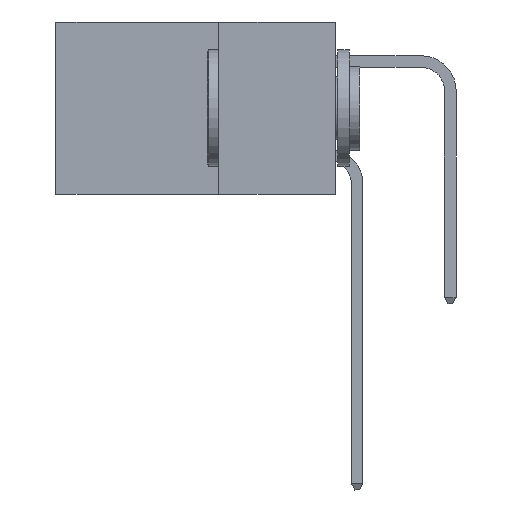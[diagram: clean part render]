
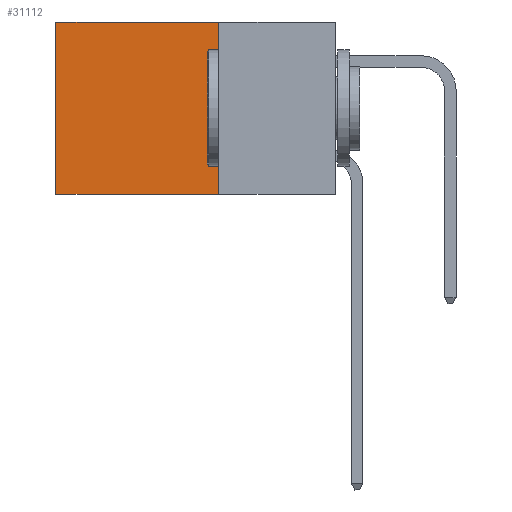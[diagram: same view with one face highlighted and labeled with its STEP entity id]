
A CAD part, left-side view. The second image highlights one B-rep face of the part: STEP entity #31112.
In plain terms, the highlighted planar face has unit normal (-1, 0, 0).
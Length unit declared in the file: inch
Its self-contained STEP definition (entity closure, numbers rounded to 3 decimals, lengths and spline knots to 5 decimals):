
#366 = DIRECTION ( 'NONE',  ( 0., 0., -1. ) ) ;
#1197 = CARTESIAN_POINT ( 'NONE',  ( 0.2875, 0.25, 0. ) ) ;
#2785 = PLANE ( 'NONE',  #10819 ) ;
#3038 = EDGE_CURVE ( 'NONE', #17193, #27264, #29164, .T. ) ;
#5011 = CARTESIAN_POINT ( 'NONE',  ( 0.2875, 0.25, -0.37 ) ) ;
#5106 = VECTOR ( 'NONE', #8847, 39.37008 ) ;
#6699 = CARTESIAN_POINT ( 'NONE',  ( 0.2875, 0.25, 0. ) ) ;
#6942 = EDGE_LOOP ( 'NONE', ( #30878, #9580, #10173, #22482 ) ) ;
#7513 = LINE ( 'NONE', #6699, #21998 ) ;
#7831 = CARTESIAN_POINT ( 'NONE',  ( 0.2875, 0.6, 0. ) ) ;
#8000 = CARTESIAN_POINT ( 'NONE',  ( 0.2875, 0.25, 0. ) ) ;
#8847 = DIRECTION ( 'NONE',  ( 0., 1., 0. ) ) ;
#9580 = ORIENTED_EDGE ( 'NONE', *, *, #3038, .F. ) ;
#10173 = ORIENTED_EDGE ( 'NONE', *, *, #23232, .F. ) ;
#10225 = DIRECTION ( 'NONE',  ( 0., 0., -1. ) ) ;
#10819 = AXIS2_PLACEMENT_3D ( 'NONE', #8000, #33164, #10225 ) ;
#10913 = CARTESIAN_POINT ( 'NONE',  ( 0.2875, 0.25, 0. ) ) ;
#11859 = EDGE_CURVE ( 'NONE', #25325, #27370, #22038, .T. ) ;
#13449 = CARTESIAN_POINT ( 'NONE',  ( 0.2875, 0.6, 0. ) ) ;
#17193 = VERTEX_POINT ( 'NONE', #30893 ) ;
#18094 = VECTOR ( 'NONE', #366, 39.37008 ) ;
#20544 = EDGE_CURVE ( 'NONE', #27370, #27264, #24944, .T. ) ;
#21998 = VECTOR ( 'NONE', #26725, 39.37008 ) ;
#22038 = LINE ( 'NONE', #1197, #5106 ) ;
#22482 = ORIENTED_EDGE ( 'NONE', *, *, #11859, .T. ) ;
#22989 = DIRECTION ( 'NONE',  ( 0., 1., 0. ) ) ;
#23232 = EDGE_CURVE ( 'NONE', #25325, #17193, #7513, .T. ) ;
#23350 = FACE_OUTER_BOUND ( 'NONE', #6942, .T. ) ;
#24944 = LINE ( 'NONE', #13449, #18094 ) ;
#25325 = VERTEX_POINT ( 'NONE', #10913 ) ;
#26725 = DIRECTION ( 'NONE',  ( 0., 0., -1. ) ) ;
#27264 = VERTEX_POINT ( 'NONE', #30645 ) ;
#27370 = VERTEX_POINT ( 'NONE', #7831 ) ;
#28729 = VECTOR ( 'NONE', #22989, 39.37008 ) ;
#29164 = LINE ( 'NONE', #5011, #28729 ) ;
#30645 = CARTESIAN_POINT ( 'NONE',  ( 0.2875, 0.6, -0.37 ) ) ;
#30878 = ORIENTED_EDGE ( 'NONE', *, *, #20544, .T. ) ;
#30893 = CARTESIAN_POINT ( 'NONE',  ( 0.2875, 0.25, -0.37 ) ) ;
#31112 = ADVANCED_FACE ( 'NONE', ( #23350 ), #2785, .F. ) ;
#33164 = DIRECTION ( 'NONE',  ( 1., 0., 0. ) ) ;
